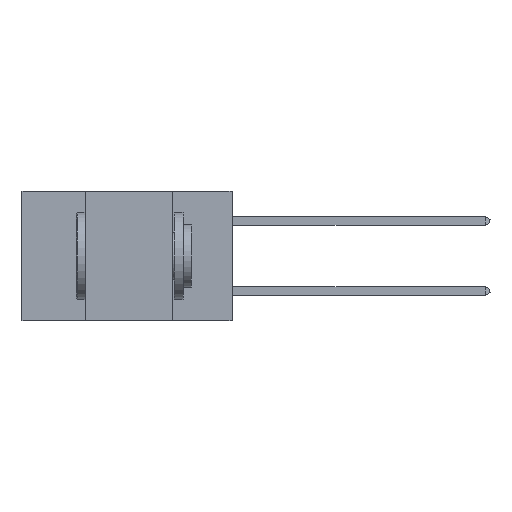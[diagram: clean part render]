
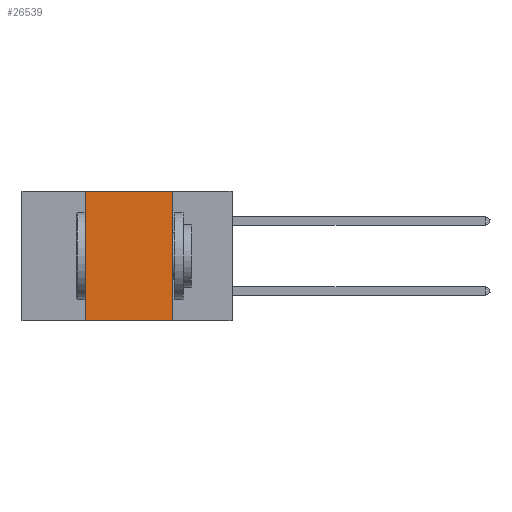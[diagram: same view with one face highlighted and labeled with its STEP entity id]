
A CAD part, left-side view. The second image highlights one B-rep face of the part: STEP entity #26539.
In plain terms, the highlighted planar face has unit normal (-1, 0, 0).
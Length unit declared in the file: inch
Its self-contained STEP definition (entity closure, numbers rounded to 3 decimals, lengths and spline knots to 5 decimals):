
#577 = CARTESIAN_POINT ( 'NONE',  ( 0., 0.42, 0. ) ) ;
#772 = VERTEX_POINT ( 'NONE', #577 ) ;
#1517 = ORIENTED_EDGE ( 'NONE', *, *, #46311, .F. ) ;
#8710 = LINE ( 'NONE', #33250, #21255 ) ;
#10118 = VERTEX_POINT ( 'NONE', #42680 ) ;
#10345 = EDGE_CURVE ( 'NONE', #41484, #772, #8710, .T. ) ;
#10768 = CARTESIAN_POINT ( 'NONE',  ( 0., 0.17, 0. ) ) ;
#11101 = EDGE_CURVE ( 'NONE', #21437, #10118, #29152, .T. ) ;
#12128 = VECTOR ( 'NONE', #22176, 39.37008 ) ;
#14110 = LINE ( 'NONE', #33360, #15811 ) ;
#15811 = VECTOR ( 'NONE', #18697, 39.37008 ) ;
#16273 = CARTESIAN_POINT ( 'NONE',  ( 0., 0.42, -0.37 ) ) ;
#16751 = DIRECTION ( 'NONE',  ( 1., 0., 0. ) ) ;
#18697 = DIRECTION ( 'NONE',  ( 0., -1., 0. ) ) ;
#18847 = DIRECTION ( 'NONE',  ( 0., 0., -1. ) ) ;
#18887 = ORIENTED_EDGE ( 'NONE', *, *, #10345, .F. ) ;
#20418 = CARTESIAN_POINT ( 'NONE',  ( 0., 0.6, 0. ) ) ;
#20563 = PLANE ( 'NONE',  #25548 ) ;
#21255 = VECTOR ( 'NONE', #26100, 39.37008 ) ;
#21437 = VERTEX_POINT ( 'NONE', #10768 ) ;
#22176 = DIRECTION ( 'NONE',  ( 0., -1., 0. ) ) ;
#25548 = AXIS2_PLACEMENT_3D ( 'NONE', #20418, #16751, #27268 ) ;
#26100 = DIRECTION ( 'NONE',  ( 0., 0., 1. ) ) ;
#26539 = ADVANCED_FACE ( 'NONE', ( #40916 ), #20563, .F. ) ;
#27268 = DIRECTION ( 'NONE',  ( 0., 0., -1. ) ) ;
#29152 = LINE ( 'NONE', #37190, #43446 ) ;
#33250 = CARTESIAN_POINT ( 'NONE',  ( 0., 0.42, 0. ) ) ;
#33360 = CARTESIAN_POINT ( 'NONE',  ( 0., 0.6, -0.37 ) ) ;
#34532 = EDGE_LOOP ( 'NONE', ( #41554, #1517, #18887, #45397 ) ) ;
#37190 = CARTESIAN_POINT ( 'NONE',  ( 0., 0.17, 0. ) ) ;
#37624 = EDGE_CURVE ( 'NONE', #41484, #10118, #14110, .T. ) ;
#40520 = CARTESIAN_POINT ( 'NONE',  ( 0., 0.6, 0. ) ) ;
#40916 = FACE_OUTER_BOUND ( 'NONE', #34532, .T. ) ;
#41484 = VERTEX_POINT ( 'NONE', #16273 ) ;
#41554 = ORIENTED_EDGE ( 'NONE', *, *, #11101, .F. ) ;
#42376 = LINE ( 'NONE', #40520, #12128 ) ;
#42680 = CARTESIAN_POINT ( 'NONE',  ( 0., 0.17, -0.37 ) ) ;
#43446 = VECTOR ( 'NONE', #18847, 39.37008 ) ;
#45397 = ORIENTED_EDGE ( 'NONE', *, *, #37624, .T. ) ;
#46311 = EDGE_CURVE ( 'NONE', #772, #21437, #42376, .T. ) ;
